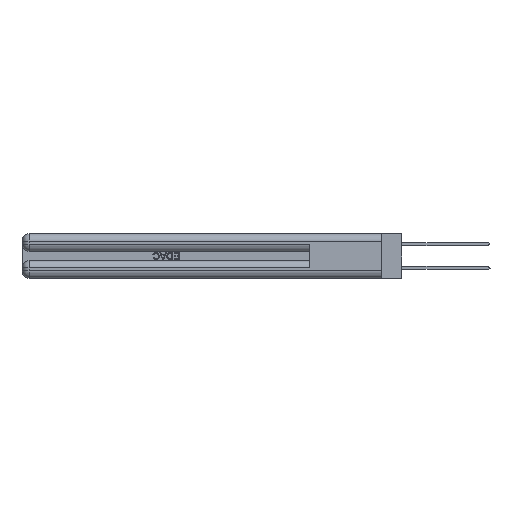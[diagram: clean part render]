
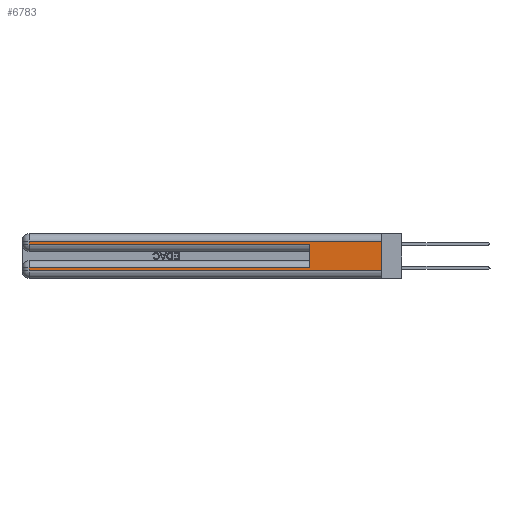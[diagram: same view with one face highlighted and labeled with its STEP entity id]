
A CAD part, left-side view. The second image highlights one B-rep face of the part: STEP entity #6783.
In plain terms, the highlighted planar face has unit normal (-1, 0, 0).
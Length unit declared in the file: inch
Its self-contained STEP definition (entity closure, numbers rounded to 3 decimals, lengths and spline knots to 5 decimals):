
#728 = CARTESIAN_POINT ( 'NONE',  ( 0., 0.6, 0.145 ) ) ;
#1093 = LINE ( 'NONE', #31080, #36310 ) ;
#2013 = ORIENTED_EDGE ( 'NONE', *, *, #8175, .F. ) ;
#3704 = DIRECTION ( 'NONE',  ( 0., -1., 0. ) ) ;
#3897 = EDGE_CURVE ( 'NONE', #19994, #9834, #15768, .T. ) ;
#4063 = LINE ( 'NONE', #41523, #20637 ) ;
#4424 = VERTEX_POINT ( 'NONE', #5033 ) ;
#4833 = VECTOR ( 'NONE', #19521, 39.37008 ) ;
#5033 = CARTESIAN_POINT ( 'NONE',  ( 0., 2.94, 0.31 ) ) ;
#5881 = CARTESIAN_POINT ( 'NONE',  ( 0., 2.94, 0.37 ) ) ;
#6210 = DIRECTION ( 'NONE',  ( 0., 0., -1. ) ) ;
#6478 = VECTOR ( 'NONE', #18162, 39.37008 ) ;
#6727 = CARTESIAN_POINT ( 'NONE',  ( 0., 0., 0.37 ) ) ;
#6783 = ADVANCED_FACE ( 'NONE', ( #16128 ), #13255, .F. ) ;
#7075 = LINE ( 'NONE', #26552, #4833 ) ;
#7197 = LINE ( 'NONE', #6727, #26404 ) ;
#7823 = EDGE_CURVE ( 'NONE', #26807, #17506, #1093, .T. ) ;
#7998 = VECTOR ( 'NONE', #34234, 39.37008 ) ;
#8175 = EDGE_CURVE ( 'NONE', #8851, #17506, #7197, .T. ) ;
#8230 = ORIENTED_EDGE ( 'NONE', *, *, #43427, .T. ) ;
#8851 = VERTEX_POINT ( 'NONE', #37047 ) ;
#8983 = ORIENTED_EDGE ( 'NONE', *, *, #3897, .T. ) ;
#9732 = VECTOR ( 'NONE', #13800, 39.37008 ) ;
#9834 = VERTEX_POINT ( 'NONE', #28136 ) ;
#13131 = CARTESIAN_POINT ( 'NONE',  ( 0., 0., 0.06 ) ) ;
#13255 = PLANE ( 'NONE',  #42239 ) ;
#13800 = DIRECTION ( 'NONE',  ( 0., -1., 0. ) ) ;
#15768 = LINE ( 'NONE', #16917, #9732 ) ;
#16128 = FACE_OUTER_BOUND ( 'NONE', #24282, .T. ) ;
#16546 = EDGE_CURVE ( 'NONE', #8851, #4424, #7075, .T. ) ;
#16917 = CARTESIAN_POINT ( 'NONE',  ( 0., 0., 0.285 ) ) ;
#17506 = VERTEX_POINT ( 'NONE', #13131 ) ;
#17636 = ORIENTED_EDGE ( 'NONE', *, *, #7823, .T. ) ;
#18162 = DIRECTION ( 'NONE',  ( 0., 0., 1. ) ) ;
#19521 = DIRECTION ( 'NONE',  ( 0., 1., 0. ) ) ;
#19994 = VERTEX_POINT ( 'NONE', #30393 ) ;
#20037 = DIRECTION ( 'NONE',  ( 1., 0., 0. ) ) ;
#20385 = CARTESIAN_POINT ( 'NONE',  ( 0., 2.94, 0.06 ) ) ;
#20407 = EDGE_CURVE ( 'NONE', #30855, #26807, #30390, .T. ) ;
#20556 = DIRECTION ( 'NONE',  ( 0., 0., -1. ) ) ;
#20637 = VECTOR ( 'NONE', #44919, 39.37008 ) ;
#22643 = CARTESIAN_POINT ( 'NONE',  ( 0., 0.6, 0.085 ) ) ;
#24282 = EDGE_LOOP ( 'NONE', ( #2013, #34264, #8230, #8983, #39642, #43918, #34257, #17636 ) ) ;
#26404 = VECTOR ( 'NONE', #27901, 39.37008 ) ;
#26552 = CARTESIAN_POINT ( 'NONE',  ( 0., 0., 0.31 ) ) ;
#26807 = VERTEX_POINT ( 'NONE', #20385 ) ;
#27901 = DIRECTION ( 'NONE',  ( 0., 0., -1. ) ) ;
#28136 = CARTESIAN_POINT ( 'NONE',  ( 0., 0.6, 0.285 ) ) ;
#30390 = LINE ( 'NONE', #38601, #32517 ) ;
#30393 = CARTESIAN_POINT ( 'NONE',  ( 0., 2.94, 0.285 ) ) ;
#30855 = VERTEX_POINT ( 'NONE', #32677 ) ;
#31080 = CARTESIAN_POINT ( 'NONE',  ( 0., 0., 0.06 ) ) ;
#32228 = LINE ( 'NONE', #728, #6478 ) ;
#32517 = VECTOR ( 'NONE', #20556, 39.37008 ) ;
#32677 = CARTESIAN_POINT ( 'NONE',  ( 0., 2.94, 0.085 ) ) ;
#34234 = DIRECTION ( 'NONE',  ( 0., 0., -1. ) ) ;
#34257 = ORIENTED_EDGE ( 'NONE', *, *, #20407, .T. ) ;
#34264 = ORIENTED_EDGE ( 'NONE', *, *, #16546, .T. ) ;
#34266 = CARTESIAN_POINT ( 'NONE',  ( 0., 0., 0.37 ) ) ;
#35644 = VERTEX_POINT ( 'NONE', #22643 ) ;
#36310 = VECTOR ( 'NONE', #3704, 39.37008 ) ;
#37047 = CARTESIAN_POINT ( 'NONE',  ( 0., 0., 0.31 ) ) ;
#38601 = CARTESIAN_POINT ( 'NONE',  ( 0., 2.94, 0.37 ) ) ;
#39191 = EDGE_CURVE ( 'NONE', #35644, #9834, #32228, .T. ) ;
#39642 = ORIENTED_EDGE ( 'NONE', *, *, #39191, .F. ) ;
#40713 = EDGE_CURVE ( 'NONE', #35644, #30855, #4063, .T. ) ;
#40969 = LINE ( 'NONE', #5881, #7998 ) ;
#41523 = CARTESIAN_POINT ( 'NONE',  ( 0., 0., 0.085 ) ) ;
#42239 = AXIS2_PLACEMENT_3D ( 'NONE', #34266, #20037, #6210 ) ;
#43427 = EDGE_CURVE ( 'NONE', #4424, #19994, #40969, .T. ) ;
#43918 = ORIENTED_EDGE ( 'NONE', *, *, #40713, .T. ) ;
#44919 = DIRECTION ( 'NONE',  ( 0., 1., 0. ) ) ;
